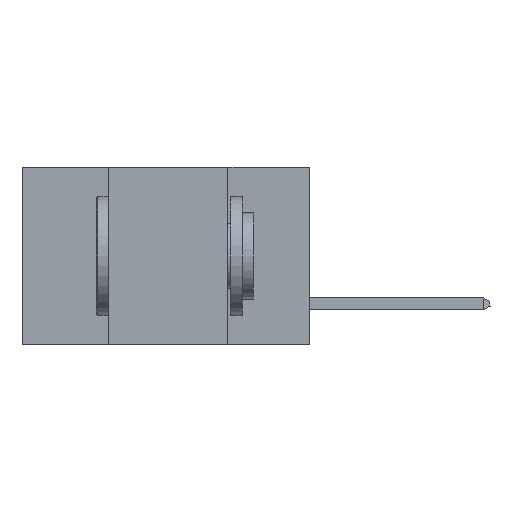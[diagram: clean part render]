
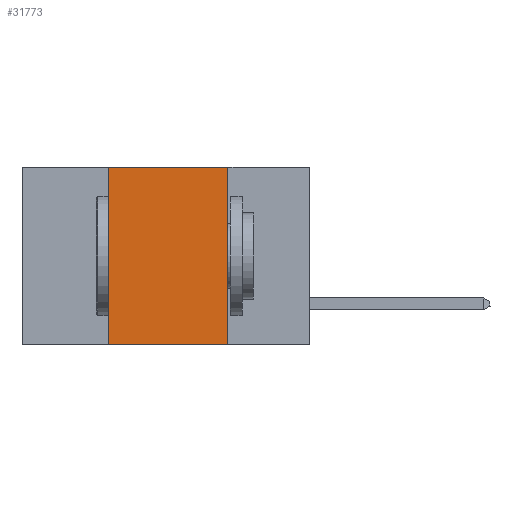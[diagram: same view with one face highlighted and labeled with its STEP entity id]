
A CAD part, left-side view. The second image highlights one B-rep face of the part: STEP entity #31773.
In plain terms, the highlighted planar face has unit normal (-1, 0, 0).
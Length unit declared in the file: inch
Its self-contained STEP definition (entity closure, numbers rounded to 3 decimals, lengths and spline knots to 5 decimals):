
#3321 = VERTEX_POINT ( 'NONE', #31424 ) ;
#7378 = ORIENTED_EDGE ( 'NONE', *, *, #16343, .F. ) ;
#10189 = VECTOR ( 'NONE', #32538, 39.37008 ) ;
#10256 = CARTESIAN_POINT ( 'NONE',  ( 0., 0.6, 0. ) ) ;
#10524 = EDGE_CURVE ( 'NONE', #3321, #23493, #32647, .T. ) ;
#11177 = VERTEX_POINT ( 'NONE', #39860 ) ;
#11680 = VERTEX_POINT ( 'NONE', #39256 ) ;
#13566 = CARTESIAN_POINT ( 'NONE',  ( 0., 0.42, 0. ) ) ;
#13861 = DIRECTION ( 'NONE',  ( 0., 0., -1. ) ) ;
#16343 = EDGE_CURVE ( 'NONE', #23493, #11177, #35554, .T. ) ;
#17556 = CARTESIAN_POINT ( 'NONE',  ( 0., 0.42, 0. ) ) ;
#19767 = DIRECTION ( 'NONE',  ( 0., 0., -1. ) ) ;
#19796 = FACE_OUTER_BOUND ( 'NONE', #23362, .T. ) ;
#20581 = EDGE_CURVE ( 'NONE', #11177, #11680, #37155, .T. ) ;
#21394 = DIRECTION ( 'NONE',  ( 0., -1., 0. ) ) ;
#21845 = ORIENTED_EDGE ( 'NONE', *, *, #35045, .T. ) ;
#22824 = PLANE ( 'NONE',  #36852 ) ;
#23362 = EDGE_LOOP ( 'NONE', ( #40393, #7378, #29863, #21845 ) ) ;
#23493 = VERTEX_POINT ( 'NONE', #17556 ) ;
#28744 = VECTOR ( 'NONE', #13861, 39.37008 ) ;
#29352 = CARTESIAN_POINT ( 'NONE',  ( 0., 0.6, -0.37 ) ) ;
#29604 = DIRECTION ( 'NONE',  ( 0., 0., 1. ) ) ;
#29863 = ORIENTED_EDGE ( 'NONE', *, *, #10524, .F. ) ;
#31367 = CARTESIAN_POINT ( 'NONE',  ( 0., 0.6, 0. ) ) ;
#31424 = CARTESIAN_POINT ( 'NONE',  ( 0., 0.42, -0.37 ) ) ;
#31773 = ADVANCED_FACE ( 'NONE', ( #19796 ), #22824, .F. ) ;
#32538 = DIRECTION ( 'NONE',  ( 0., -1., 0. ) ) ;
#32647 = LINE ( 'NONE', #13566, #33642 ) ;
#33642 = VECTOR ( 'NONE', #29604, 39.37008 ) ;
#34068 = VECTOR ( 'NONE', #21394, 39.37008 ) ;
#35045 = EDGE_CURVE ( 'NONE', #3321, #11680, #35452, .T. ) ;
#35452 = LINE ( 'NONE', #29352, #10189 ) ;
#35554 = LINE ( 'NONE', #31367, #34068 ) ;
#36852 = AXIS2_PLACEMENT_3D ( 'NONE', #10256, #38759, #19767 ) ;
#37155 = LINE ( 'NONE', #39609, #28744 ) ;
#38759 = DIRECTION ( 'NONE',  ( 1., 0., 0. ) ) ;
#39256 = CARTESIAN_POINT ( 'NONE',  ( 0., 0.17, -0.37 ) ) ;
#39609 = CARTESIAN_POINT ( 'NONE',  ( 0., 0.17, 0. ) ) ;
#39860 = CARTESIAN_POINT ( 'NONE',  ( 0., 0.17, 0. ) ) ;
#40393 = ORIENTED_EDGE ( 'NONE', *, *, #20581, .F. ) ;
